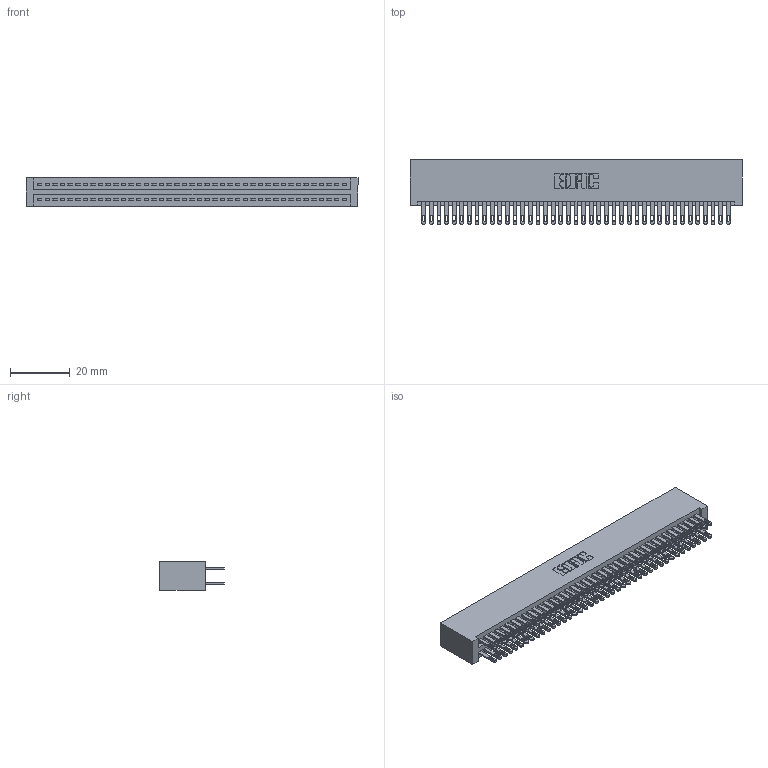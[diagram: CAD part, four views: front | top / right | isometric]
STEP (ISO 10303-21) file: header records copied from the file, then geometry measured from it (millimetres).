
FILE_DESCRIPTION (( 'STEP AP203' ), '1' );
FILE_NAME ('345-082-500-201.STEP', '2018-10-03T20:46:52', ( '' ), ( '' ), 'SwSTEP 2.0', 'SolidWorks 2016', '' );
FILE_SCHEMA (( 'CONFIG_CONTROL_DESIGN' ));
Length unit declared in the file: inch
Products named in the file (3): 345-082-500-201; 345-292-001_345-293-100; 345 Part_No Mounting Lugs
Assembly tree (83 placements, depth 2):
  345-082-500-201
    345 Part_No Mounting Lugs
    345-292-001_345-293-100  x82
Bounding box: 110.74 x 21.51 x 9.4 mm (x, y, z)
Volume: 11615 mm3; surface area: 18289.2 mm2
Topology: 83 solids, 83 shells, 3890 faces, 11879 edges, 7918 vertices
Faces by surface type: plane 2290, cylinder 1600
Entity records: 31957 total; most frequent: CARTESIAN_POINT 5356, ORIENTED_EDGE 5290, DIRECTION 4721, EDGE_CURVE 2645, VECTOR 2353, LINE 2353, VERTEX_POINT 1762, AXIS2_PLACEMENT_3D 1184
